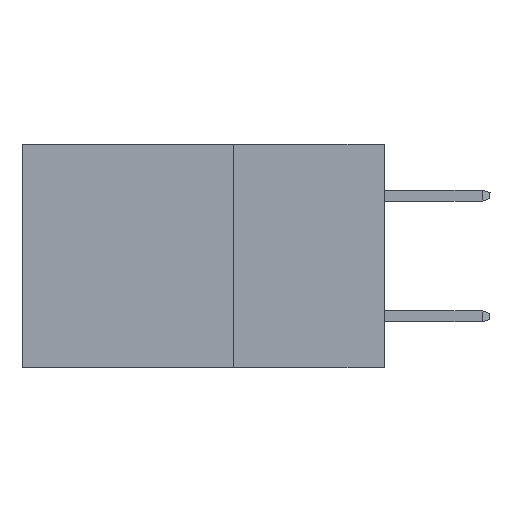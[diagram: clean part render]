
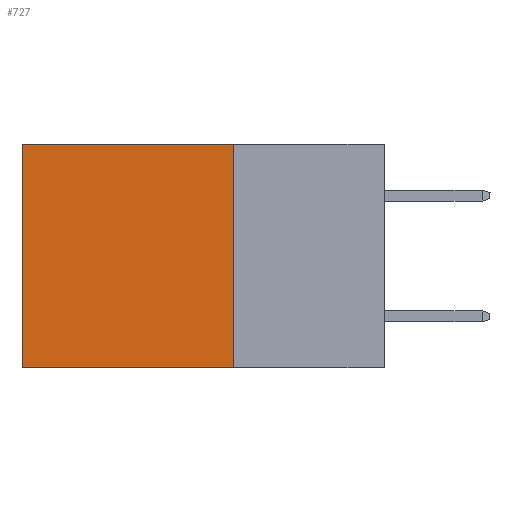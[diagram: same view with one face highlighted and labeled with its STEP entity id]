
A CAD part, left-side view. The second image highlights one B-rep face of the part: STEP entity #727.
In plain terms, the highlighted planar face has unit normal (-1, 0, 0).
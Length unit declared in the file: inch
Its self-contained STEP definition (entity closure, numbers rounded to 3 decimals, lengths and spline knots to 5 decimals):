
#64 = DIRECTION ( 'NONE',  ( 0., 1., 0. ) ) ;
#727 = ADVANCED_FACE ( 'NONE', ( #5451 ), #3466, .F. ) ;
#2139 = DIRECTION ( 'NONE',  ( 0., 0., -1. ) ) ;
#2228 = CARTESIAN_POINT ( 'NONE',  ( 0.298, 0.25, 0. ) ) ;
#2262 = VECTOR ( 'NONE', #2139, 39.37008 ) ;
#3038 = DIRECTION ( 'NONE',  ( 0., 1., 0. ) ) ;
#3044 = LINE ( 'NONE', #10363, #2262 ) ;
#3397 = CARTESIAN_POINT ( 'NONE',  ( 0.298, 0.25, 0. ) ) ;
#3466 = PLANE ( 'NONE',  #10282 ) ;
#3909 = EDGE_CURVE ( 'NONE', #7346, #5649, #7950, .T. ) ;
#5111 = LINE ( 'NONE', #2228, #10921 ) ;
#5134 = ORIENTED_EDGE ( 'NONE', *, *, #7175, .T. ) ;
#5195 = VECTOR ( 'NONE', #9540, 39.37008 ) ;
#5451 = FACE_OUTER_BOUND ( 'NONE', #6447, .T. ) ;
#5649 = VERTEX_POINT ( 'NONE', #12396 ) ;
#5664 = VERTEX_POINT ( 'NONE', #9293 ) ;
#5765 = LINE ( 'NONE', #9192, #9161 ) ;
#6407 = CARTESIAN_POINT ( 'NONE',  ( 0.298, 0.25, 0. ) ) ;
#6447 = EDGE_LOOP ( 'NONE', ( #5134, #13109, #13002, #7252 ) ) ;
#6712 = EDGE_CURVE ( 'NONE', #5649, #5664, #5765, .T. ) ;
#7175 = EDGE_CURVE ( 'NONE', #13260, #5664, #3044, .T. ) ;
#7252 = ORIENTED_EDGE ( 'NONE', *, *, #10245, .T. ) ;
#7346 = VERTEX_POINT ( 'NONE', #3397 ) ;
#7505 = CARTESIAN_POINT ( 'NONE',  ( 0.298, 0.25, 0. ) ) ;
#7950 = LINE ( 'NONE', #6407, #5195 ) ;
#8830 = CARTESIAN_POINT ( 'NONE',  ( 0.298, 0.6, 0. ) ) ;
#9161 = VECTOR ( 'NONE', #3038, 39.37008 ) ;
#9192 = CARTESIAN_POINT ( 'NONE',  ( 0.298, 0.25, -0.37 ) ) ;
#9293 = CARTESIAN_POINT ( 'NONE',  ( 0.298, 0.6, -0.37 ) ) ;
#9540 = DIRECTION ( 'NONE',  ( 0., 0., -1. ) ) ;
#10245 = EDGE_CURVE ( 'NONE', #7346, #13260, #5111, .T. ) ;
#10282 = AXIS2_PLACEMENT_3D ( 'NONE', #7505, #10819, #12858 ) ;
#10363 = CARTESIAN_POINT ( 'NONE',  ( 0.298, 0.6, 0. ) ) ;
#10819 = DIRECTION ( 'NONE',  ( 1., 0., 0. ) ) ;
#10921 = VECTOR ( 'NONE', #64, 39.37008 ) ;
#12396 = CARTESIAN_POINT ( 'NONE',  ( 0.298, 0.25, -0.37 ) ) ;
#12858 = DIRECTION ( 'NONE',  ( 0., 0., -1. ) ) ;
#13002 = ORIENTED_EDGE ( 'NONE', *, *, #3909, .F. ) ;
#13109 = ORIENTED_EDGE ( 'NONE', *, *, #6712, .F. ) ;
#13260 = VERTEX_POINT ( 'NONE', #8830 ) ;
